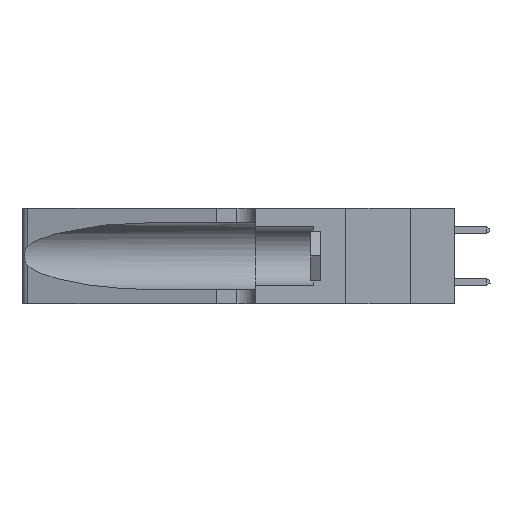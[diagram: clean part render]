
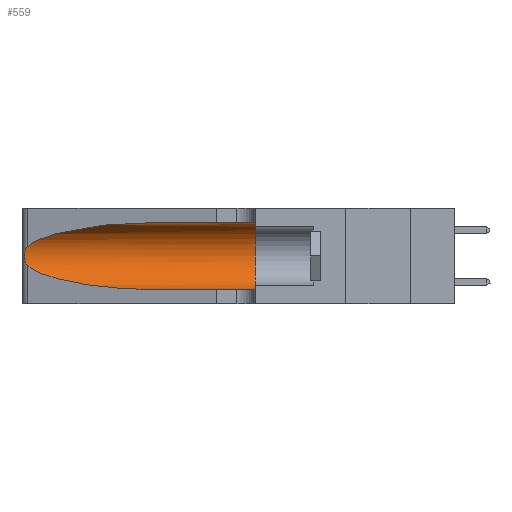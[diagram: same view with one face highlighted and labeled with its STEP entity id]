
A CAD part, left-side view. The second image highlights one B-rep face of the part: STEP entity #559.
In plain terms, the highlighted cylindrical face has radius 3.308 mm (diameter 6.617 mm), a partial arc.
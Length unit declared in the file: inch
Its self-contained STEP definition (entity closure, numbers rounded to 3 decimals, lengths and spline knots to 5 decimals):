
#39 = CARTESIAN_POINT ( 'NONE',  ( 0.2373, 1.15595, 0.28018 ) ) ;
#559 = ADVANCED_FACE ( 'NONE', ( #12015 ), #3372, .F. ) ;
#609 = CARTESIAN_POINT ( 'NONE',  ( 0.25555, 1.22994, 0.2215 ) ) ;
#685 = CARTESIAN_POINT ( 'NONE',  ( 0.25856, 1.23593, 0.16098 ) ) ;
#977 = EDGE_CURVE ( 'NONE', #11411, #13145, #12454, .T. ) ;
#1047 = DIRECTION ( 'NONE',  ( 0., 1., 0. ) ) ;
#1165 = DIRECTION ( 'NONE',  ( 0., -1., 0. ) ) ;
#1889 = CARTESIAN_POINT ( 'NONE',  ( 0.1305, 0.72297, 0.05475 ) ) ;
#1966 = VERTEX_POINT ( 'NONE', #2585 ) ;
#1991 = EDGE_CURVE ( 'NONE', #11411, #1966, #11236, .T. ) ;
#2156 = VERTEX_POINT ( 'NONE', #6185 ) ;
#2246 = CARTESIAN_POINT ( 'NONE',  ( 0.25639, 1.23186, 0.15144 ) ) ;
#2585 = CARTESIAN_POINT ( 'NONE',  ( 0.25487, 1.22718, 0.22369 ) ) ;
#3372 = CYLINDRICAL_SURFACE ( 'NONE', #8922, 0.13025 ) ;
#3839 = CARTESIAN_POINT ( 'NONE',  ( 0.25487, 1.22718, 0.14631 ) ) ;
#4255 = ORIENTED_EDGE ( 'NONE', *, *, #18718, .T. ) ;
#4410 = ORIENTED_EDGE ( 'NONE', *, *, #14071, .T. ) ;
#4931 = CARTESIAN_POINT ( 'NONE',  ( 0.2373, 1.15595, 0.08982 ) ) ;
#4987 = CARTESIAN_POINT ( 'NONE',  ( 0.25487, 1.22718, 0.14631 ) ) ;
#5050 = VERTEX_POINT ( 'NONE', #6070 ) ;
#5266 = CARTESIAN_POINT ( 'NONE',  ( 0.25487, 1.22718, 0.22369 ) ) ;
#5328 = CARTESIAN_POINT ( 'NONE',  ( 0.25639, 1.23184, 0.21858 ) ) ;
#5529 = CARTESIAN_POINT ( 'NONE',  ( 0.1305, 0.72297, 0.31525 ) ) ;
#5876 = CARTESIAN_POINT ( 'NONE',  ( 0.18966, 0.96281, 0.31525 ) ) ;
#6070 = CARTESIAN_POINT ( 'NONE',  ( 0.25487, 1.22718, 0.14631 ) ) ;
#6159 = CARTESIAN_POINT ( 'NONE',  ( 0.1305, 1.61858, 0.05475 ) ) ;
#6185 = CARTESIAN_POINT ( 'NONE',  ( 0.1305, 0.35, 0.05475 ) ) ;
#6470 = EDGE_CURVE ( 'NONE', #10665, #2156, #11042, .T. ) ;
#6908 = CARTESIAN_POINT ( 'NONE',  ( 0.25854, 1.2359, 0.20912 ) ) ;
#6978 = ORIENTED_EDGE ( 'NONE', *, *, #1991, .T. ) ;
#7460 = CARTESIAN_POINT ( 'NONE',  ( 0.1305, 1.61858, 0.31525 ) ) ;
#8223 = CARTESIAN_POINT ( 'NONE',  ( 0.1305, 0.35, 0.31525 ) ) ;
#8401 = CARTESIAN_POINT ( 'NONE',  ( 0.1305, 0.72297, 0.31525 ) ) ;
#8427 = CARTESIAN_POINT ( 'NONE',  ( 0.26075, 1.23896, 0.19203 ) ) ;
#8922 = AXIS2_PLACEMENT_3D ( 'NONE', #15996, #16078, #14879 ) ;
#9548 = AXIS2_PLACEMENT_3D ( 'NONE', #10351, #1047, #11832 ) ;
#9995 = CARTESIAN_POINT ( 'NONE',  ( 0.26017, 1.23833, 0.17102 ) ) ;
#10351 = CARTESIAN_POINT ( 'NONE',  ( 0.1305, 0.35, 0.185 ) ) ;
#10411 = ORIENTED_EDGE ( 'NONE', *, *, #6470, .T. ) ;
#10665 = VERTEX_POINT ( 'NONE', #15820 ) ;
#10932 = ORIENTED_EDGE ( 'NONE', *, *, #18256, .F. ) ;
#11042 = LINE ( 'NONE', #6159, #18446 ) ;
#11148 = CARTESIAN_POINT ( 'NONE',  ( 0.18966, 0.96281, 0.05475 ) ) ;
#11216 = CIRCLE ( 'NONE', #9548, 0.13025 ) ;
#11236 =( BOUNDED_CURVE ( )  B_SPLINE_CURVE ( 3, ( #8401, #5876, #39, #17126 ),
 .UNSPECIFIED., .F., .T. ) 
 B_SPLINE_CURVE_WITH_KNOTS ( ( 4, 4 ),
 ( 1.5708, 2.84003 ),
 .UNSPECIFIED. ) 
 CURVE ( )  GEOMETRIC_REPRESENTATION_ITEM ( )  RATIONAL_B_SPLINE_CURVE ( ( 1., 0.87, 0.87, 1. ) ) 
 REPRESENTATION_ITEM ( '' )  );
#11411 = VERTEX_POINT ( 'NONE', #5529 ) ;
#11475 = CARTESIAN_POINT ( 'NONE',  ( 0.25789, 1.23486, 0.15765 ) ) ;
#11832 = DIRECTION ( 'NONE',  ( 0., 0., 1. ) ) ;
#12015 = FACE_OUTER_BOUND ( 'NONE', #19543, .T. ) ;
#12262 = DIRECTION ( 'NONE',  ( 0., -1., 0. ) ) ;
#12454 = LINE ( 'NONE', #7460, #17791 ) ;
#12662 = ORIENTED_EDGE ( 'NONE', *, *, #977, .F. ) ;
#12978 = CARTESIAN_POINT ( 'NONE',  ( 0.25555, 1.22993, 0.14849 ) ) ;
#13129 = B_SPLINE_CURVE_WITH_KNOTS ( 'NONE', 3,
 ( #5266, #609, #5328, #15867, #6908, #17377, #8427, #18853, #9995, #685, #11475, #2246, #12978, #3839 ),
 .UNSPECIFIED., .F., .F.,
 ( 4, 2, 2, 2, 2, 2, 4 ),
 ( 0., 0.00027, 0.00053, 0.00107, 0.0016, 0.00187, 0.00214 ),
 .UNSPECIFIED. ) ;
#13145 = VERTEX_POINT ( 'NONE', #8223 ) ;
#13662 =( BOUNDED_CURVE ( )  B_SPLINE_CURVE ( 3, ( #4987, #4931, #11148, #1889 ),
 .UNSPECIFIED., .F., .F. ) 
 B_SPLINE_CURVE_WITH_KNOTS ( ( 4, 4 ),
 ( 3.44316, 4.71239 ),
 .UNSPECIFIED. ) 
 CURVE ( )  GEOMETRIC_REPRESENTATION_ITEM ( )  RATIONAL_B_SPLINE_CURVE ( ( 1., 0.87, 0.87, 1. ) ) 
 REPRESENTATION_ITEM ( '' )  );
#14071 = EDGE_CURVE ( 'NONE', #5050, #10665, #13662, .T. ) ;
#14879 = DIRECTION ( 'NONE',  ( 0., 0., -1. ) ) ;
#15820 = CARTESIAN_POINT ( 'NONE',  ( 0.1305, 0.72297, 0.05475 ) ) ;
#15867 = CARTESIAN_POINT ( 'NONE',  ( 0.25787, 1.23484, 0.2124 ) ) ;
#15996 = CARTESIAN_POINT ( 'NONE',  ( 0.1305, 1.61858, 0.185 ) ) ;
#16078 = DIRECTION ( 'NONE',  ( 0., -1., 0. ) ) ;
#17126 = CARTESIAN_POINT ( 'NONE',  ( 0.25487, 1.22718, 0.22369 ) ) ;
#17377 = CARTESIAN_POINT ( 'NONE',  ( 0.26018, 1.23835, 0.19895 ) ) ;
#17791 = VECTOR ( 'NONE', #1165, 39.37008 ) ;
#18256 = EDGE_CURVE ( 'NONE', #13145, #2156, #11216, .T. ) ;
#18446 = VECTOR ( 'NONE', #12262, 39.37008 ) ;
#18718 = EDGE_CURVE ( 'NONE', #1966, #5050, #13129, .T. ) ;
#18853 = CARTESIAN_POINT ( 'NONE',  ( 0.26075, 1.23896, 0.178 ) ) ;
#19543 = EDGE_LOOP ( 'NONE', ( #6978, #4255, #4410, #10411, #10932, #12662 ) ) ;
